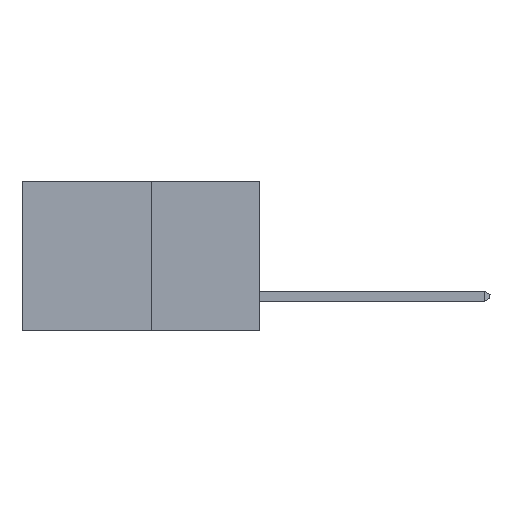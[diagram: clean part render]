
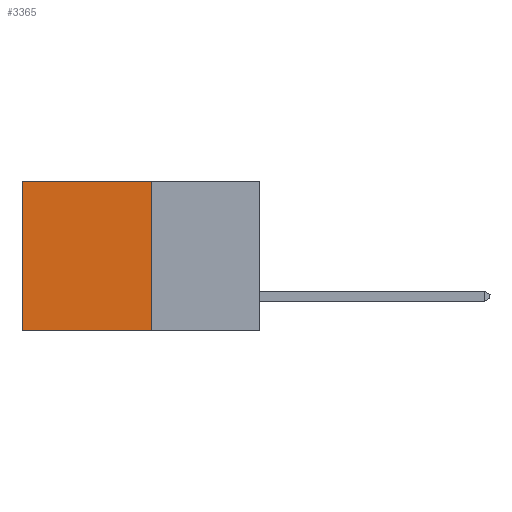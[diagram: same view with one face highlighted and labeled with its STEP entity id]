
A CAD part, left-side view. The second image highlights one B-rep face of the part: STEP entity #3365.
In plain terms, the highlighted planar face has unit normal (-1, 0, 0).
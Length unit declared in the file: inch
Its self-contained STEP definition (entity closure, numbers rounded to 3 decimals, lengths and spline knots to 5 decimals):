
#180 = ORIENTED_EDGE ( 'NONE', *, *, #6508, .T. ) ;
#352 = CARTESIAN_POINT ( 'NONE',  ( 0.277, 0.59, -0.37 ) ) ;
#749 = DIRECTION ( 'NONE',  ( 0., 0., -1. ) ) ;
#1218 = VECTOR ( 'NONE', #2771, 39.37008 ) ;
#1637 = DIRECTION ( 'NONE',  ( 0., 0., -1. ) ) ;
#1676 = DIRECTION ( 'NONE',  ( 1., 0., 0. ) ) ;
#1720 = PLANE ( 'NONE',  #7603 ) ;
#1781 = CARTESIAN_POINT ( 'NONE',  ( 0.277, 0.27, 0. ) ) ;
#2157 = CARTESIAN_POINT ( 'NONE',  ( 0.277, 0.27, -0.37 ) ) ;
#2248 = CARTESIAN_POINT ( 'NONE',  ( 0.277, 0.27, -0.37 ) ) ;
#2528 = ORIENTED_EDGE ( 'NONE', *, *, #11288, .F. ) ;
#2739 = EDGE_CURVE ( 'NONE', #11694, #7465, #2988, .T. ) ;
#2771 = DIRECTION ( 'NONE',  ( 0., 1., 0. ) ) ;
#2893 = EDGE_LOOP ( 'NONE', ( #180, #12116, #2528, #5654 ) ) ;
#2988 = LINE ( 'NONE', #12351, #5323 ) ;
#3365 = ADVANCED_FACE ( 'NONE', ( #8830 ), #1720, .F. ) ;
#3758 = CARTESIAN_POINT ( 'NONE',  ( 0.277, 0.27, -0.37 ) ) ;
#5063 = CARTESIAN_POINT ( 'NONE',  ( 0.277, 0.59, -0.37 ) ) ;
#5131 = CARTESIAN_POINT ( 'NONE',  ( 0.277, 0.27, 0. ) ) ;
#5323 = VECTOR ( 'NONE', #5453, 39.37008 ) ;
#5453 = DIRECTION ( 'NONE',  ( 0., 1., 0. ) ) ;
#5594 = VECTOR ( 'NONE', #6272, 39.37008 ) ;
#5654 = ORIENTED_EDGE ( 'NONE', *, *, #12640, .T. ) ;
#6272 = DIRECTION ( 'NONE',  ( 0., 0., -1. ) ) ;
#6508 = EDGE_CURVE ( 'NONE', #8569, #7465, #8470, .T. ) ;
#7465 = VERTEX_POINT ( 'NONE', #5063 ) ;
#7603 = AXIS2_PLACEMENT_3D ( 'NONE', #2248, #1676, #1637 ) ;
#8375 = VECTOR ( 'NONE', #749, 39.37008 ) ;
#8470 = LINE ( 'NONE', #352, #5594 ) ;
#8569 = VERTEX_POINT ( 'NONE', #11768 ) ;
#8830 = FACE_OUTER_BOUND ( 'NONE', #2893, .T. ) ;
#9093 = LINE ( 'NONE', #1781, #1218 ) ;
#10877 = VERTEX_POINT ( 'NONE', #5131 ) ;
#10915 = LINE ( 'NONE', #3758, #8375 ) ;
#11288 = EDGE_CURVE ( 'NONE', #10877, #11694, #10915, .T. ) ;
#11694 = VERTEX_POINT ( 'NONE', #2157 ) ;
#11768 = CARTESIAN_POINT ( 'NONE',  ( 0.277, 0.59, 0. ) ) ;
#12116 = ORIENTED_EDGE ( 'NONE', *, *, #2739, .F. ) ;
#12351 = CARTESIAN_POINT ( 'NONE',  ( 0.277, 0.27, -0.37 ) ) ;
#12640 = EDGE_CURVE ( 'NONE', #10877, #8569, #9093, .T. ) ;
